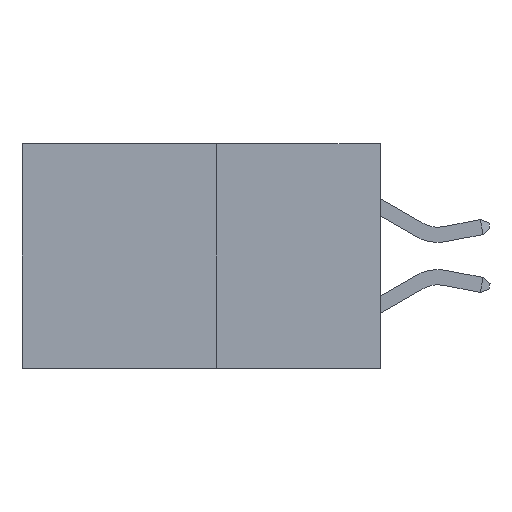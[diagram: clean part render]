
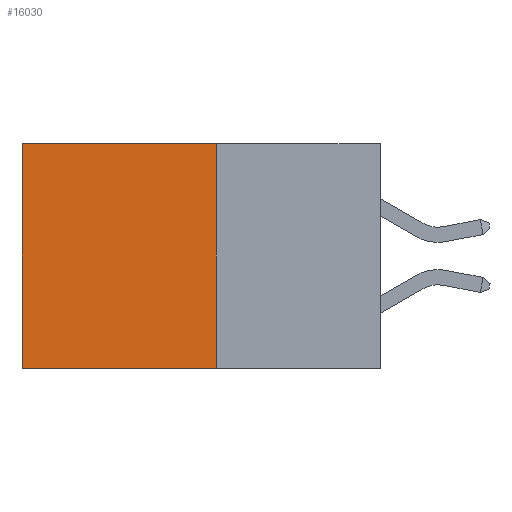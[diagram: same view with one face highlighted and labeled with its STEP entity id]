
A CAD part, left-side view. The second image highlights one B-rep face of the part: STEP entity #16030.
In plain terms, the highlighted planar face has unit normal (-1, 0, 0).
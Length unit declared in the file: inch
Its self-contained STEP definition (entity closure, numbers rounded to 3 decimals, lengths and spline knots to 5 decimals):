
#617 = CARTESIAN_POINT ( 'NONE',  ( 0.277, 0.59, 0. ) ) ;
#1350 = LINE ( 'NONE', #11240, #12478 ) ;
#1626 = CARTESIAN_POINT ( 'NONE',  ( 0.277, 0.27, -0.37 ) ) ;
#1933 = ORIENTED_EDGE ( 'NONE', *, *, #15568, .F. ) ;
#3281 = ORIENTED_EDGE ( 'NONE', *, *, #4051, .F. ) ;
#4051 = EDGE_CURVE ( 'NONE', #7533, #17735, #16128, .T. ) ;
#4492 = DIRECTION ( 'NONE',  ( 1., 0., 0. ) ) ;
#5006 = FACE_OUTER_BOUND ( 'NONE', #6468, .T. ) ;
#5022 = VECTOR ( 'NONE', #10368, 39.37008 ) ;
#5023 = VECTOR ( 'NONE', #14426, 39.37008 ) ;
#5834 = PLANE ( 'NONE',  #9877 ) ;
#6468 = EDGE_LOOP ( 'NONE', ( #11884, #1933, #3281, #6495 ) ) ;
#6495 = ORIENTED_EDGE ( 'NONE', *, *, #10835, .T. ) ;
#6961 = VECTOR ( 'NONE', #16885, 39.37008 ) ;
#7533 = VERTEX_POINT ( 'NONE', #10364 ) ;
#8259 = CARTESIAN_POINT ( 'NONE',  ( 0.277, 0.27, -0.37 ) ) ;
#9232 = CARTESIAN_POINT ( 'NONE',  ( 0.277, 0.59, -0.37 ) ) ;
#9877 = AXIS2_PLACEMENT_3D ( 'NONE', #10035, #4492, #14246 ) ;
#9908 = CARTESIAN_POINT ( 'NONE',  ( 0.277, 0.59, -0.37 ) ) ;
#10035 = CARTESIAN_POINT ( 'NONE',  ( 0.277, 0.27, -0.37 ) ) ;
#10364 = CARTESIAN_POINT ( 'NONE',  ( 0.277, 0.27, 0. ) ) ;
#10368 = DIRECTION ( 'NONE',  ( 0., 0., -1. ) ) ;
#10835 = EDGE_CURVE ( 'NONE', #7533, #11112, #1350, .T. ) ;
#11112 = VERTEX_POINT ( 'NONE', #617 ) ;
#11121 = LINE ( 'NONE', #9908, #6961 ) ;
#11240 = CARTESIAN_POINT ( 'NONE',  ( 0.277, 0.27, 0. ) ) ;
#11706 = CARTESIAN_POINT ( 'NONE',  ( 0.277, 0.27, -0.37 ) ) ;
#11884 = ORIENTED_EDGE ( 'NONE', *, *, #12991, .T. ) ;
#12015 = LINE ( 'NONE', #11706, #5023 ) ;
#12478 = VECTOR ( 'NONE', #15347, 39.37008 ) ;
#12991 = EDGE_CURVE ( 'NONE', #11112, #17558, #11121, .T. ) ;
#14246 = DIRECTION ( 'NONE',  ( 0., 0., -1. ) ) ;
#14426 = DIRECTION ( 'NONE',  ( 0., 1., 0. ) ) ;
#15347 = DIRECTION ( 'NONE',  ( 0., 1., 0. ) ) ;
#15568 = EDGE_CURVE ( 'NONE', #17735, #17558, #12015, .T. ) ;
#16030 = ADVANCED_FACE ( 'NONE', ( #5006 ), #5834, .F. ) ;
#16128 = LINE ( 'NONE', #1626, #5022 ) ;
#16885 = DIRECTION ( 'NONE',  ( 0., 0., -1. ) ) ;
#17558 = VERTEX_POINT ( 'NONE', #9232 ) ;
#17735 = VERTEX_POINT ( 'NONE', #8259 ) ;
